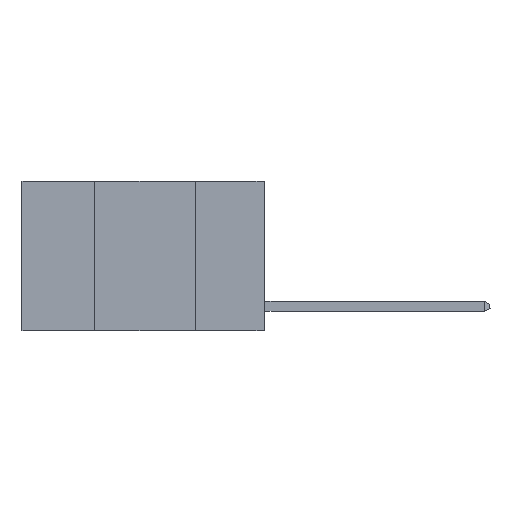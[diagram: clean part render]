
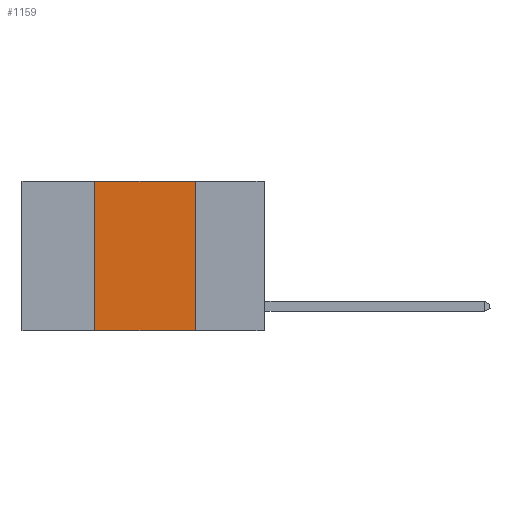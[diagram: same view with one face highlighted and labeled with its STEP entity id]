
A CAD part, left-side view. The second image highlights one B-rep face of the part: STEP entity #1159.
In plain terms, the highlighted planar face has unit normal (-1, 0, 0).
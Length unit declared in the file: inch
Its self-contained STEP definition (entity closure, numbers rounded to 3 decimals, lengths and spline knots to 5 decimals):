
#954 = LINE ( 'NONE', #2326, #6259 ) ;
#1091 = CARTESIAN_POINT ( 'NONE',  ( 0., 0.6, -0.37 ) ) ;
#1159 = ADVANCED_FACE ( 'NONE', ( #10991 ), #10759, .F. ) ;
#1172 = DIRECTION ( 'NONE',  ( 0., -1., 0. ) ) ;
#1957 = EDGE_CURVE ( 'NONE', #15846, #11085, #10255, .T. ) ;
#2326 = CARTESIAN_POINT ( 'NONE',  ( 0., 0.42, 0. ) ) ;
#3112 = LINE ( 'NONE', #8018, #4524 ) ;
#3505 = DIRECTION ( 'NONE',  ( 1., 0., 0. ) ) ;
#4524 = VECTOR ( 'NONE', #13942, 39.37008 ) ;
#5580 = AXIS2_PLACEMENT_3D ( 'NONE', #7300, #3505, #11974 ) ;
#6251 = CARTESIAN_POINT ( 'NONE',  ( 0., 0.17, 0. ) ) ;
#6259 = VECTOR ( 'NONE', #13449, 39.37008 ) ;
#7300 = CARTESIAN_POINT ( 'NONE',  ( 0., 0.6, 0. ) ) ;
#7308 = LINE ( 'NONE', #1091, #8605 ) ;
#7511 = ORIENTED_EDGE ( 'NONE', *, *, #1957, .F. ) ;
#8018 = CARTESIAN_POINT ( 'NONE',  ( 0., 0.17, 0. ) ) ;
#8381 = VERTEX_POINT ( 'NONE', #14816 ) ;
#8605 = VECTOR ( 'NONE', #1172, 39.37008 ) ;
#9032 = DIRECTION ( 'NONE',  ( 0., -1., 0. ) ) ;
#9639 = ORIENTED_EDGE ( 'NONE', *, *, #13680, .F. ) ;
#9845 = CARTESIAN_POINT ( 'NONE',  ( 0., 0.42, -0.37 ) ) ;
#10013 = VECTOR ( 'NONE', #9032, 39.37008 ) ;
#10255 = LINE ( 'NONE', #10417, #10013 ) ;
#10417 = CARTESIAN_POINT ( 'NONE',  ( 0., 0.6, 0. ) ) ;
#10759 = PLANE ( 'NONE',  #5580 ) ;
#10908 = EDGE_CURVE ( 'NONE', #11085, #8381, #3112, .T. ) ;
#10991 = FACE_OUTER_BOUND ( 'NONE', #13540, .T. ) ;
#11085 = VERTEX_POINT ( 'NONE', #6251 ) ;
#11974 = DIRECTION ( 'NONE',  ( 0., 0., -1. ) ) ;
#12870 = CARTESIAN_POINT ( 'NONE',  ( 0., 0.42, 0. ) ) ;
#13322 = VERTEX_POINT ( 'NONE', #9845 ) ;
#13449 = DIRECTION ( 'NONE',  ( 0., 0., 1. ) ) ;
#13540 = EDGE_LOOP ( 'NONE', ( #14403, #7511, #9639, #15828 ) ) ;
#13680 = EDGE_CURVE ( 'NONE', #13322, #15846, #954, .T. ) ;
#13942 = DIRECTION ( 'NONE',  ( 0., 0., -1. ) ) ;
#14211 = EDGE_CURVE ( 'NONE', #13322, #8381, #7308, .T. ) ;
#14403 = ORIENTED_EDGE ( 'NONE', *, *, #10908, .F. ) ;
#14816 = CARTESIAN_POINT ( 'NONE',  ( 0., 0.17, -0.37 ) ) ;
#15828 = ORIENTED_EDGE ( 'NONE', *, *, #14211, .T. ) ;
#15846 = VERTEX_POINT ( 'NONE', #12870 ) ;
